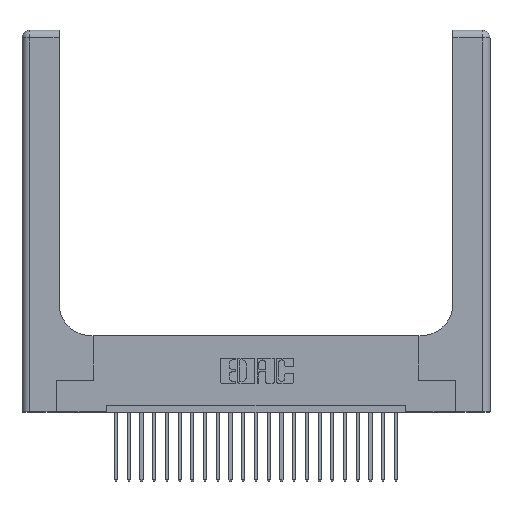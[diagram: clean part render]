
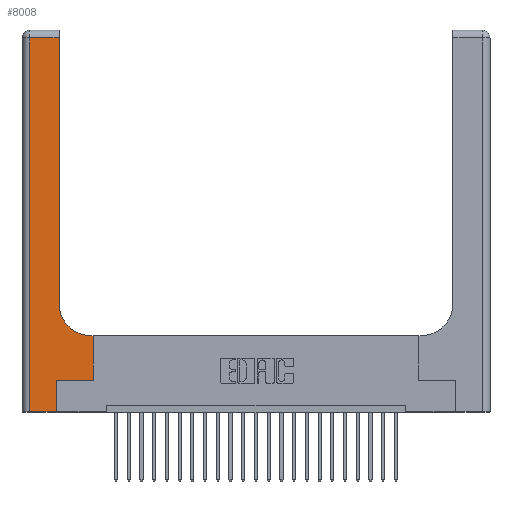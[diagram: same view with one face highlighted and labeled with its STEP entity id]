
A CAD part, top view. The second image highlights one B-rep face of the part: STEP entity #8008.
In plain terms, the highlighted planar face has unit normal (0, 0, 1).
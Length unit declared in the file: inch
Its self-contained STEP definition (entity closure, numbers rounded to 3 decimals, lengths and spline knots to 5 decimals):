
#153 = CARTESIAN_POINT ( 'NONE',  ( 0.269, 0.25, 0.37 ) ) ;
#765 = CARTESIAN_POINT ( 'NONE',  ( 0.5415, 0.6, 0.37 ) ) ;
#1149 = EDGE_CURVE ( 'NONE', #21215, #19207, #10116, .T. ) ;
#1254 = DIRECTION ( 'NONE',  ( 0., 1., 0. ) ) ;
#1256 = VECTOR ( 'NONE', #3570, 39.37008 ) ;
#1267 = PLANE ( 'NONE',  #14924 ) ;
#1428 = ORIENTED_EDGE ( 'NONE', *, *, #1149, .T. ) ;
#1861 = ORIENTED_EDGE ( 'NONE', *, *, #22375, .T. ) ;
#2164 = CARTESIAN_POINT ( 'NONE',  ( 0.5585, 0.6, 0.37 ) ) ;
#2377 = EDGE_CURVE ( 'NONE', #6796, #10911, #2454, .T. ) ;
#2454 = LINE ( 'NONE', #19700, #24233 ) ;
#2991 = CARTESIAN_POINT ( 'NONE',  ( 0.5415, 0.85, 0.37 ) ) ;
#2996 = DIRECTION ( 'NONE',  ( 0., 1., 0. ) ) ;
#3403 = LINE ( 'NONE', #22031, #10710 ) ;
#3570 = DIRECTION ( 'NONE',  ( -1., 0., 0. ) ) ;
#4442 = FACE_OUTER_BOUND ( 'NONE', #17099, .T. ) ;
#5148 = DIRECTION ( 'NONE',  ( -1., 0., 0. ) ) ;
#5618 = VERTEX_POINT ( 'NONE', #765 ) ;
#5778 = VERTEX_POINT ( 'NONE', #153 ) ;
#6392 = AXIS2_PLACEMENT_3D ( 'NONE', #2991, #6795, #8613 ) ;
#6733 = VECTOR ( 'NONE', #1254, 39.37008 ) ;
#6795 = DIRECTION ( 'NONE',  ( 0., 0., -1. ) ) ;
#6796 = VERTEX_POINT ( 'NONE', #20271 ) ;
#6861 = CARTESIAN_POINT ( 'NONE',  ( 0.269, 0., 0.37 ) ) ;
#7188 = CARTESIAN_POINT ( 'NONE',  ( 0.269, 0., 0.37 ) ) ;
#8008 = ADVANCED_FACE ( 'NONE', ( #4442 ), #1267, .F. ) ;
#8613 = DIRECTION ( 'NONE',  ( 1., 0., 0. ) ) ;
#8723 = DIRECTION ( 'NONE',  ( 0., -1., 0. ) ) ;
#8738 = CARTESIAN_POINT ( 'NONE',  ( 0.2915, 3., 0.37 ) ) ;
#8924 = CARTESIAN_POINT ( 'NONE',  ( 0., 3., 0.37 ) ) ;
#9244 = ORIENTED_EDGE ( 'NONE', *, *, #2377, .T. ) ;
#9410 = VERTEX_POINT ( 'NONE', #12996 ) ;
#10116 = LINE ( 'NONE', #8738, #14930 ) ;
#10501 = CIRCLE ( 'NONE', #6392, 0.25 ) ;
#10710 = VECTOR ( 'NONE', #21876, 39.37008 ) ;
#10911 = VERTEX_POINT ( 'NONE', #2164 ) ;
#11853 = CARTESIAN_POINT ( 'NONE',  ( 0.2915, 2.94, 0.37 ) ) ;
#11925 = VERTEX_POINT ( 'NONE', #21979 ) ;
#12282 = VERTEX_POINT ( 'NONE', #6861 ) ;
#12575 = LINE ( 'NONE', #19252, #17078 ) ;
#12784 = ORIENTED_EDGE ( 'NONE', *, *, #15193, .T. ) ;
#12996 = CARTESIAN_POINT ( 'NONE',  ( 0.06, 0., 0.37 ) ) ;
#14924 = AXIS2_PLACEMENT_3D ( 'NONE', #8924, #16586, #5148 ) ;
#14930 = VECTOR ( 'NONE', #24667, 39.37008 ) ;
#15165 = CARTESIAN_POINT ( 'NONE',  ( 0.2915, 0.6, 0.37 ) ) ;
#15193 = EDGE_CURVE ( 'NONE', #12282, #5778, #17307, .T. ) ;
#15208 = DIRECTION ( 'NONE',  ( -1., 0., 0. ) ) ;
#16586 = DIRECTION ( 'NONE',  ( 0., 0., -1. ) ) ;
#16824 = ORIENTED_EDGE ( 'NONE', *, *, #23472, .T. ) ;
#17078 = VECTOR ( 'NONE', #21028, 39.37008 ) ;
#17099 = EDGE_LOOP ( 'NONE', ( #1428, #23744, #19334, #1861, #12784, #16824, #9244, #22137, #23262 ) ) ;
#17307 = LINE ( 'NONE', #7188, #6733 ) ;
#18512 = LINE ( 'NONE', #23148, #24529 ) ;
#19141 = VECTOR ( 'NONE', #8723, 39.37008 ) ;
#19207 = VERTEX_POINT ( 'NONE', #11853 ) ;
#19252 = CARTESIAN_POINT ( 'NONE',  ( 0., 0., 0.37 ) ) ;
#19334 = ORIENTED_EDGE ( 'NONE', *, *, #24640, .T. ) ;
#19700 = CARTESIAN_POINT ( 'NONE',  ( 0.5585, 0.25, 0.37 ) ) ;
#20271 = CARTESIAN_POINT ( 'NONE',  ( 0.5585, 0.25, 0.37 ) ) ;
#20364 = LINE ( 'NONE', #21731, #19141 ) ;
#21028 = DIRECTION ( 'NONE',  ( 1., 0., 0. ) ) ;
#21215 = VERTEX_POINT ( 'NONE', #23045 ) ;
#21527 = EDGE_CURVE ( 'NONE', #5618, #21215, #10501, .T. ) ;
#21731 = CARTESIAN_POINT ( 'NONE',  ( 0.06, 3., 0.37 ) ) ;
#21876 = DIRECTION ( 'NONE',  ( 1., 0., 0. ) ) ;
#21979 = CARTESIAN_POINT ( 'NONE',  ( 0.06, 2.94, 0.37 ) ) ;
#22031 = CARTESIAN_POINT ( 'NONE',  ( 0.269, 0.25, 0.37 ) ) ;
#22137 = ORIENTED_EDGE ( 'NONE', *, *, #23703, .T. ) ;
#22375 = EDGE_CURVE ( 'NONE', #9410, #12282, #12575, .T. ) ;
#23045 = CARTESIAN_POINT ( 'NONE',  ( 0.2915, 0.85, 0.37 ) ) ;
#23047 = LINE ( 'NONE', #15165, #1256 ) ;
#23148 = CARTESIAN_POINT ( 'NONE',  ( 0., 2.94, 0.37 ) ) ;
#23262 = ORIENTED_EDGE ( 'NONE', *, *, #21527, .T. ) ;
#23472 = EDGE_CURVE ( 'NONE', #5778, #6796, #3403, .T. ) ;
#23703 = EDGE_CURVE ( 'NONE', #10911, #5618, #23047, .T. ) ;
#23744 = ORIENTED_EDGE ( 'NONE', *, *, #24264, .T. ) ;
#24233 = VECTOR ( 'NONE', #2996, 39.37008 ) ;
#24264 = EDGE_CURVE ( 'NONE', #19207, #11925, #18512, .T. ) ;
#24529 = VECTOR ( 'NONE', #15208, 39.37008 ) ;
#24640 = EDGE_CURVE ( 'NONE', #11925, #9410, #20364, .T. ) ;
#24667 = DIRECTION ( 'NONE',  ( 0., 1., 0. ) ) ;
